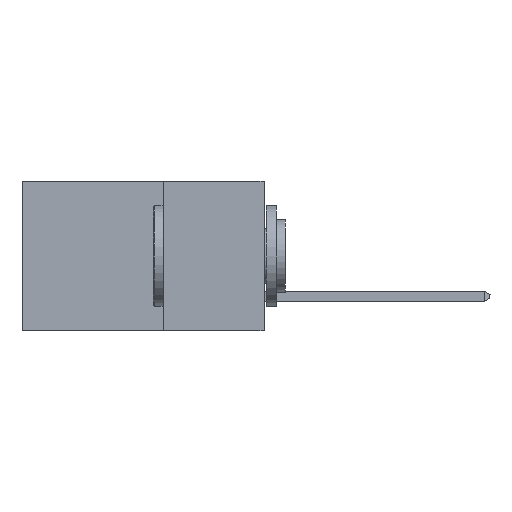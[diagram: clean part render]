
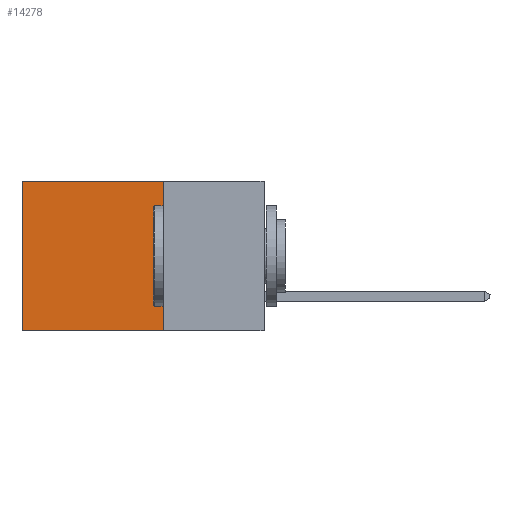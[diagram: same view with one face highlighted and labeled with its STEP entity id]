
A CAD part, left-side view. The second image highlights one B-rep face of the part: STEP entity #14278.
In plain terms, the highlighted planar face has unit normal (-1, 0, 0).
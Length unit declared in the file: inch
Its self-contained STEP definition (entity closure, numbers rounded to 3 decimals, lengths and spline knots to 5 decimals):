
#164 = EDGE_CURVE ( 'NONE', #11804, #8099, #8557, .T. ) ;
#912 = PLANE ( 'NONE',  #5999 ) ;
#1833 = EDGE_CURVE ( 'NONE', #16958, #3985, #16641, .T. ) ;
#2222 = VECTOR ( 'NONE', #8649, 39.37008 ) ;
#2761 = CARTESIAN_POINT ( 'NONE',  ( 0.2615, 0.6, -0.37 ) ) ;
#3045 = DIRECTION ( 'NONE',  ( 0., 1., 0. ) ) ;
#3683 = CARTESIAN_POINT ( 'NONE',  ( 0.2615, 0.25, -0.37 ) ) ;
#3985 = VERTEX_POINT ( 'NONE', #19583 ) ;
#4199 = CARTESIAN_POINT ( 'NONE',  ( 0.2615, 0.25, -0.37 ) ) ;
#5677 = DIRECTION ( 'NONE',  ( 1., 0., 0. ) ) ;
#5999 = AXIS2_PLACEMENT_3D ( 'NONE', #4199, #5677, #16004 ) ;
#7575 = ORIENTED_EDGE ( 'NONE', *, *, #164, .F. ) ;
#8099 = VERTEX_POINT ( 'NONE', #18919 ) ;
#8557 = LINE ( 'NONE', #14597, #17574 ) ;
#8649 = DIRECTION ( 'NONE',  ( 0., 0., -1. ) ) ;
#8805 = DIRECTION ( 'NONE',  ( 0., 0., -1. ) ) ;
#9645 = LINE ( 'NONE', #3683, #2222 ) ;
#11158 = EDGE_CURVE ( 'NONE', #16958, #11804, #9645, .T. ) ;
#11480 = EDGE_LOOP ( 'NONE', ( #16049, #7575, #12051, #12315 ) ) ;
#11774 = CARTESIAN_POINT ( 'NONE',  ( 0.2615, 0.25, 0. ) ) ;
#11804 = VERTEX_POINT ( 'NONE', #15254 ) ;
#12051 = ORIENTED_EDGE ( 'NONE', *, *, #11158, .F. ) ;
#12315 = ORIENTED_EDGE ( 'NONE', *, *, #1833, .T. ) ;
#12365 = VECTOR ( 'NONE', #8805, 39.37008 ) ;
#13099 = DIRECTION ( 'NONE',  ( 0., 1., 0. ) ) ;
#13341 = VECTOR ( 'NONE', #3045, 39.37008 ) ;
#13647 = CARTESIAN_POINT ( 'NONE',  ( 0.2615, 0.25, 0. ) ) ;
#14278 = ADVANCED_FACE ( 'NONE', ( #18891 ), #912, .F. ) ;
#14597 = CARTESIAN_POINT ( 'NONE',  ( 0.2615, 0.25, -0.37 ) ) ;
#15254 = CARTESIAN_POINT ( 'NONE',  ( 0.2615, 0.25, -0.37 ) ) ;
#16004 = DIRECTION ( 'NONE',  ( 0., 0., -1. ) ) ;
#16049 = ORIENTED_EDGE ( 'NONE', *, *, #18305, .T. ) ;
#16355 = LINE ( 'NONE', #2761, #12365 ) ;
#16641 = LINE ( 'NONE', #13647, #13341 ) ;
#16958 = VERTEX_POINT ( 'NONE', #11774 ) ;
#17574 = VECTOR ( 'NONE', #13099, 39.37008 ) ;
#18305 = EDGE_CURVE ( 'NONE', #3985, #8099, #16355, .T. ) ;
#18891 = FACE_OUTER_BOUND ( 'NONE', #11480, .T. ) ;
#18919 = CARTESIAN_POINT ( 'NONE',  ( 0.2615, 0.6, -0.37 ) ) ;
#19583 = CARTESIAN_POINT ( 'NONE',  ( 0.2615, 0.6, 0. ) ) ;
